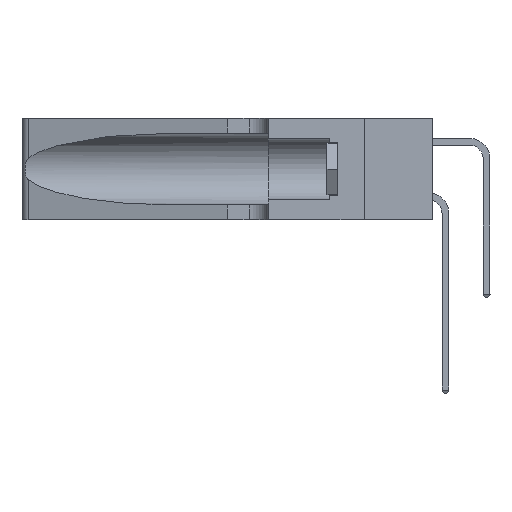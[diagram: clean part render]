
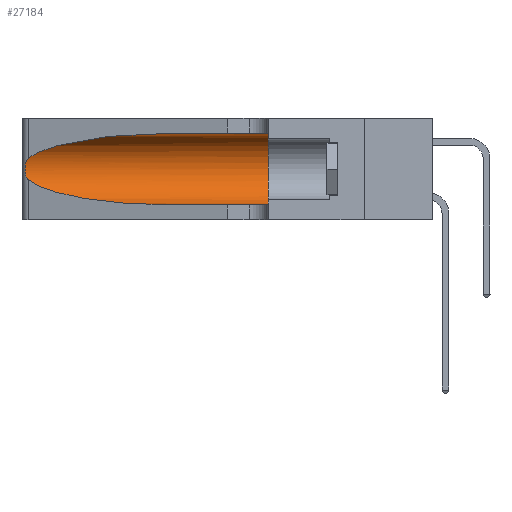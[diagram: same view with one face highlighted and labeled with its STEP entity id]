
A CAD part, left-side view. The second image highlights one B-rep face of the part: STEP entity #27184.
In plain terms, the highlighted cylindrical face has radius 3.308 mm (diameter 6.617 mm), a partial arc.
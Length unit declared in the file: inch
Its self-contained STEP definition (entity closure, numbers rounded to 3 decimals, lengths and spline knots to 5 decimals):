
#637 = EDGE_CURVE ( 'NONE', #21894, #16151, #21923, .T. ) ;
#1119 = CARTESIAN_POINT ( 'NONE',  ( 0.25639, 1.23186, 0.15144 ) ) ;
#1159 = CARTESIAN_POINT ( 'NONE',  ( 0.25487, 1.22718, 0.22369 ) ) ;
#1215 = ORIENTED_EDGE ( 'NONE', *, *, #21829, .T. ) ;
#1994 = CARTESIAN_POINT ( 'NONE',  ( 0.2373, 1.15595, 0.08982 ) ) ;
#2204 = CARTESIAN_POINT ( 'NONE',  ( 0.1305, 0.72297, 0.05475 ) ) ;
#2428 = CARTESIAN_POINT ( 'NONE',  ( 0.25487, 1.22718, 0.14631 ) ) ;
#3573 = CARTESIAN_POINT ( 'NONE',  ( 0.25789, 1.23486, 0.15765 ) ) ;
#3669 = CARTESIAN_POINT ( 'NONE',  ( 0.1305, 0.35, 0.185 ) ) ;
#3700 = LINE ( 'NONE', #9630, #22789 ) ;
#3849 = CARTESIAN_POINT ( 'NONE',  ( 0.26017, 1.23833, 0.17102 ) ) ;
#3894 = CARTESIAN_POINT ( 'NONE',  ( 0.26018, 1.23835, 0.19895 ) ) ;
#4529 = CARTESIAN_POINT ( 'NONE',  ( 0.18966, 0.96281, 0.05475 ) ) ;
#5041 = CARTESIAN_POINT ( 'NONE',  ( 0.25555, 1.22993, 0.14849 ) ) ;
#5505 =( BOUNDED_CURVE ( )  B_SPLINE_CURVE ( 3, ( #2428, #1994, #4529, #2204 ),
 .UNSPECIFIED., .F., .F. ) 
 B_SPLINE_CURVE_WITH_KNOTS ( ( 4, 4 ),
 ( 3.44316, 4.71239 ),
 .UNSPECIFIED. ) 
 CURVE ( )  GEOMETRIC_REPRESENTATION_ITEM ( )  RATIONAL_B_SPLINE_CURVE ( ( 1., 0.87, 0.87, 1. ) ) 
 REPRESENTATION_ITEM ( '' )  );
#5802 = CYLINDRICAL_SURFACE ( 'NONE', #15396, 0.13025 ) ;
#6021 = ORIENTED_EDGE ( 'NONE', *, *, #637, .T. ) ;
#6595 = AXIS2_PLACEMENT_3D ( 'NONE', #3669, #24051, #9024 ) ;
#6925 = VERTEX_POINT ( 'NONE', #25563 ) ;
#8029 = EDGE_CURVE ( 'NONE', #28988, #18228, #31063, .T. ) ;
#8375 = VERTEX_POINT ( 'NONE', #26998 ) ;
#9024 = DIRECTION ( 'NONE',  ( 0., 0., 1. ) ) ;
#9403 = EDGE_CURVE ( 'NONE', #6925, #16151, #11541, .T. ) ;
#9422 = CARTESIAN_POINT ( 'NONE',  ( 0.1305, 1.61858, 0.05475 ) ) ;
#9630 = CARTESIAN_POINT ( 'NONE',  ( 0.1305, 1.61858, 0.31525 ) ) ;
#10284 = VECTOR ( 'NONE', #13457, 39.37008 ) ;
#10622 = CARTESIAN_POINT ( 'NONE',  ( 0.1305, 1.61858, 0.185 ) ) ;
#10978 = CARTESIAN_POINT ( 'NONE',  ( 0.25487, 1.22718, 0.22369 ) ) ;
#11541 = CIRCLE ( 'NONE', #6595, 0.13025 ) ;
#11720 = B_SPLINE_CURVE_WITH_KNOTS ( 'NONE', 3,
 ( #1159, #18578, #23714, #31219, #16306, #3894, #16510, #12051, #3849, #26824, #3573, #1119, #5041, #27267 ),
 .UNSPECIFIED., .F., .F.,
 ( 4, 2, 2, 2, 2, 2, 4 ),
 ( 0., 0.00027, 0.00053, 0.00107, 0.0016, 0.00187, 0.00214 ),
 .UNSPECIFIED. ) ;
#12051 = CARTESIAN_POINT ( 'NONE',  ( 0.26075, 1.23896, 0.178 ) ) ;
#12402 = FACE_OUTER_BOUND ( 'NONE', #13986, .T. ) ;
#13457 = DIRECTION ( 'NONE',  ( 0., -1., 0. ) ) ;
#13986 = EDGE_LOOP ( 'NONE', ( #15045, #1215, #25698, #6021, #29406, #26391 ) ) ;
#15045 = ORIENTED_EDGE ( 'NONE', *, *, #8029, .T. ) ;
#15396 = AXIS2_PLACEMENT_3D ( 'NONE', #10622, #25510, #28046 ) ;
#15758 = CARTESIAN_POINT ( 'NONE',  ( 0.2373, 1.15595, 0.28018 ) ) ;
#16151 = VERTEX_POINT ( 'NONE', #16320 ) ;
#16306 = CARTESIAN_POINT ( 'NONE',  ( 0.25854, 1.2359, 0.20912 ) ) ;
#16320 = CARTESIAN_POINT ( 'NONE',  ( 0.1305, 0.35, 0.05475 ) ) ;
#16402 = CARTESIAN_POINT ( 'NONE',  ( 0.1305, 0.72297, 0.31525 ) ) ;
#16510 = CARTESIAN_POINT ( 'NONE',  ( 0.26075, 1.23896, 0.19203 ) ) ;
#18228 = VERTEX_POINT ( 'NONE', #10978 ) ;
#18578 = CARTESIAN_POINT ( 'NONE',  ( 0.25555, 1.22994, 0.2215 ) ) ;
#20403 = CARTESIAN_POINT ( 'NONE',  ( 0.25487, 1.22718, 0.22369 ) ) ;
#21829 = EDGE_CURVE ( 'NONE', #18228, #8375, #11720, .T. ) ;
#21894 = VERTEX_POINT ( 'NONE', #30118 ) ;
#21923 = LINE ( 'NONE', #9422, #10284 ) ;
#22789 = VECTOR ( 'NONE', #25415, 39.37008 ) ;
#23371 = EDGE_CURVE ( 'NONE', #28988, #6925, #3700, .T. ) ;
#23714 = CARTESIAN_POINT ( 'NONE',  ( 0.25639, 1.23184, 0.21858 ) ) ;
#23803 = EDGE_CURVE ( 'NONE', #8375, #21894, #5505, .T. ) ;
#24051 = DIRECTION ( 'NONE',  ( 0., 1., 0. ) ) ;
#25334 = CARTESIAN_POINT ( 'NONE',  ( 0.1305, 0.72297, 0.31525 ) ) ;
#25415 = DIRECTION ( 'NONE',  ( 0., -1., 0. ) ) ;
#25510 = DIRECTION ( 'NONE',  ( 0., -1., 0. ) ) ;
#25563 = CARTESIAN_POINT ( 'NONE',  ( 0.1305, 0.35, 0.31525 ) ) ;
#25698 = ORIENTED_EDGE ( 'NONE', *, *, #23803, .T. ) ;
#26391 = ORIENTED_EDGE ( 'NONE', *, *, #23371, .F. ) ;
#26824 = CARTESIAN_POINT ( 'NONE',  ( 0.25856, 1.23593, 0.16098 ) ) ;
#26998 = CARTESIAN_POINT ( 'NONE',  ( 0.25487, 1.22718, 0.14631 ) ) ;
#27184 = ADVANCED_FACE ( 'NONE', ( #12402 ), #5802, .F. ) ;
#27267 = CARTESIAN_POINT ( 'NONE',  ( 0.25487, 1.22718, 0.14631 ) ) ;
#27853 = CARTESIAN_POINT ( 'NONE',  ( 0.18966, 0.96281, 0.31525 ) ) ;
#28046 = DIRECTION ( 'NONE',  ( 0., 0., -1. ) ) ;
#28988 = VERTEX_POINT ( 'NONE', #16402 ) ;
#29406 = ORIENTED_EDGE ( 'NONE', *, *, #9403, .F. ) ;
#30118 = CARTESIAN_POINT ( 'NONE',  ( 0.1305, 0.72297, 0.05475 ) ) ;
#31063 =( BOUNDED_CURVE ( )  B_SPLINE_CURVE ( 3, ( #25334, #27853, #15758, #20403 ),
 .UNSPECIFIED., .F., .F. ) 
 B_SPLINE_CURVE_WITH_KNOTS ( ( 4, 4 ),
 ( 1.5708, 2.84003 ),
 .UNSPECIFIED. ) 
 CURVE ( )  GEOMETRIC_REPRESENTATION_ITEM ( )  RATIONAL_B_SPLINE_CURVE ( ( 1., 0.87, 0.87, 1. ) ) 
 REPRESENTATION_ITEM ( '' )  );
#31219 = CARTESIAN_POINT ( 'NONE',  ( 0.25787, 1.23484, 0.2124 ) ) ;
